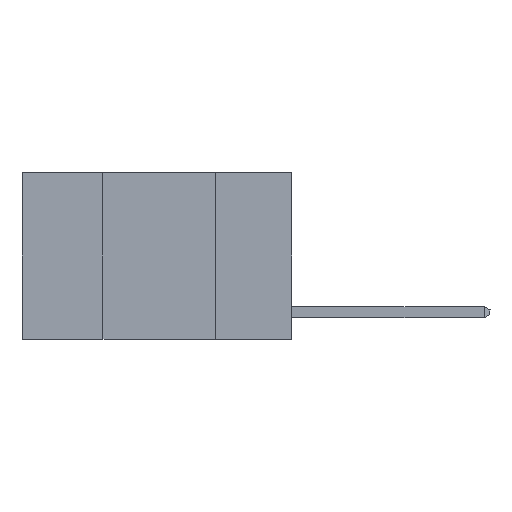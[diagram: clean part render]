
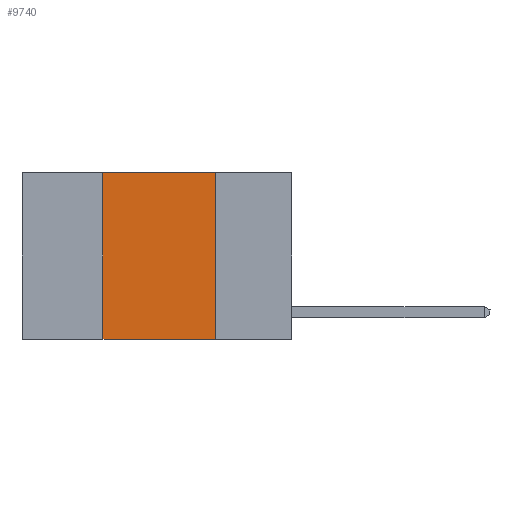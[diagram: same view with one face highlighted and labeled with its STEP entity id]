
A CAD part, left-side view. The second image highlights one B-rep face of the part: STEP entity #9740.
In plain terms, the highlighted planar face has unit normal (-1, 0, 0).
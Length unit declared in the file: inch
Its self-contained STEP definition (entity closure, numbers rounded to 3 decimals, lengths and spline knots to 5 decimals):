
#139 = DIRECTION ( 'NONE',  ( 1., 0., 0. ) ) ;
#799 = VERTEX_POINT ( 'NONE', #10735 ) ;
#1084 = DIRECTION ( 'NONE',  ( 0., 0., 1. ) ) ;
#1365 = LINE ( 'NONE', #9711, #8390 ) ;
#1558 = DIRECTION ( 'NONE',  ( 0., 0., -1. ) ) ;
#3323 = VECTOR ( 'NONE', #1084, 39.37008 ) ;
#3659 = EDGE_CURVE ( 'NONE', #12206, #10625, #8364, .T. ) ;
#4416 = DIRECTION ( 'NONE',  ( 0., -1., 0. ) ) ;
#4632 = ORIENTED_EDGE ( 'NONE', *, *, #10102, .F. ) ;
#4712 = DIRECTION ( 'NONE',  ( 0., -1., 0. ) ) ;
#5134 = EDGE_CURVE ( 'NONE', #8257, #799, #1365, .T. ) ;
#5361 = DIRECTION ( 'NONE',  ( 0., 0., -1. ) ) ;
#5728 = CARTESIAN_POINT ( 'NONE',  ( 0., 0.6, 0. ) ) ;
#5784 = EDGE_LOOP ( 'NONE', ( #5885, #12681, #4632, #7522 ) ) ;
#5885 = ORIENTED_EDGE ( 'NONE', *, *, #9176, .F. ) ;
#6390 = VECTOR ( 'NONE', #1558, 39.37008 ) ;
#7522 = ORIENTED_EDGE ( 'NONE', *, *, #5134, .T. ) ;
#7608 = CARTESIAN_POINT ( 'NONE',  ( 0., 0.42, -0.37 ) ) ;
#7797 = FACE_OUTER_BOUND ( 'NONE', #5784, .T. ) ;
#8028 = CARTESIAN_POINT ( 'NONE',  ( 0., 0.42, 0. ) ) ;
#8033 = CARTESIAN_POINT ( 'NONE',  ( 0., 0.42, 0. ) ) ;
#8257 = VERTEX_POINT ( 'NONE', #7608 ) ;
#8364 = LINE ( 'NONE', #5728, #9817 ) ;
#8390 = VECTOR ( 'NONE', #4416, 39.37008 ) ;
#8486 = CARTESIAN_POINT ( 'NONE',  ( 0., 0.6, 0. ) ) ;
#9176 = EDGE_CURVE ( 'NONE', #10625, #799, #13133, .T. ) ;
#9429 = PLANE ( 'NONE',  #10605 ) ;
#9657 = CARTESIAN_POINT ( 'NONE',  ( 0., 0.17, 0. ) ) ;
#9692 = CARTESIAN_POINT ( 'NONE',  ( 0., 0.17, 0. ) ) ;
#9711 = CARTESIAN_POINT ( 'NONE',  ( 0., 0.6, -0.37 ) ) ;
#9740 = ADVANCED_FACE ( 'NONE', ( #7797 ), #9429, .F. ) ;
#9817 = VECTOR ( 'NONE', #4712, 39.37008 ) ;
#10102 = EDGE_CURVE ( 'NONE', #8257, #12206, #10685, .T. ) ;
#10605 = AXIS2_PLACEMENT_3D ( 'NONE', #8486, #139, #5361 ) ;
#10625 = VERTEX_POINT ( 'NONE', #9657 ) ;
#10685 = LINE ( 'NONE', #8033, #3323 ) ;
#10735 = CARTESIAN_POINT ( 'NONE',  ( 0., 0.17, -0.37 ) ) ;
#12206 = VERTEX_POINT ( 'NONE', #8028 ) ;
#12681 = ORIENTED_EDGE ( 'NONE', *, *, #3659, .F. ) ;
#13133 = LINE ( 'NONE', #9692, #6390 ) ;
